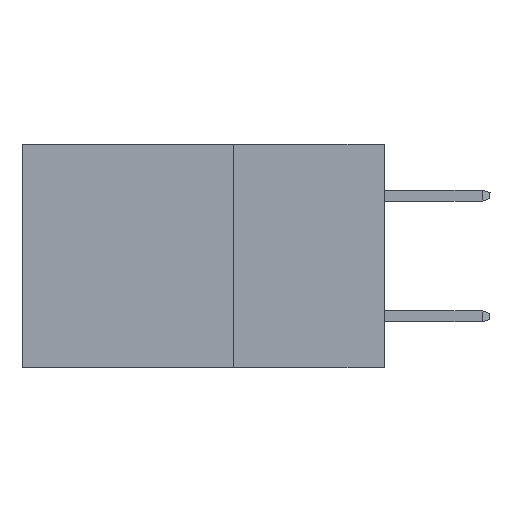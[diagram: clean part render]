
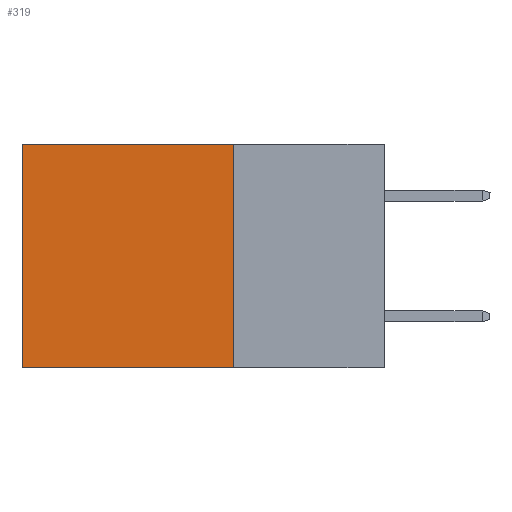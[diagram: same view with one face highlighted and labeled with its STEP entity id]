
A CAD part, left-side view. The second image highlights one B-rep face of the part: STEP entity #319.
In plain terms, the highlighted planar face has unit normal (-1, 0, 0).
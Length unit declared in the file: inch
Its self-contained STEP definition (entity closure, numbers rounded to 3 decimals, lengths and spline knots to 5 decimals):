
#319 = ADVANCED_FACE ( 'NONE', ( #1471 ), #5878, .F. ) ;
#1410 = ORIENTED_EDGE ( 'NONE', *, *, #8651, .T. ) ;
#1471 = FACE_OUTER_BOUND ( 'NONE', #7726, .T. ) ;
#1713 = DIRECTION ( 'NONE',  ( 0., 1., 0. ) ) ;
#1745 = CARTESIAN_POINT ( 'NONE',  ( 0.298, 0.6, 0. ) ) ;
#1840 = VERTEX_POINT ( 'NONE', #15833 ) ;
#2898 = DIRECTION ( 'NONE',  ( 0., 0., -1. ) ) ;
#5604 = CARTESIAN_POINT ( 'NONE',  ( 0.298, 0.25, 0. ) ) ;
#5878 = PLANE ( 'NONE',  #18901 ) ;
#6263 = CARTESIAN_POINT ( 'NONE',  ( 0.298, 0.25, -0.37 ) ) ;
#7000 = ORIENTED_EDGE ( 'NONE', *, *, #9492, .F. ) ;
#7726 = EDGE_LOOP ( 'NONE', ( #1410, #15751, #7000, #14764 ) ) ;
#7983 = VERTEX_POINT ( 'NONE', #20382 ) ;
#8651 = EDGE_CURVE ( 'NONE', #12386, #1840, #10512, .T. ) ;
#9492 = EDGE_CURVE ( 'NONE', #22242, #7983, #14454, .T. ) ;
#9864 = VECTOR ( 'NONE', #2898, 39.37008 ) ;
#10021 = LINE ( 'NONE', #18814, #10562 ) ;
#10512 = LINE ( 'NONE', #1745, #16757 ) ;
#10562 = VECTOR ( 'NONE', #20774, 39.37008 ) ;
#10763 = VECTOR ( 'NONE', #1713, 39.37008 ) ;
#10998 = CARTESIAN_POINT ( 'NONE',  ( 0.298, 0.6, 0. ) ) ;
#11555 = LINE ( 'NONE', #6263, #10763 ) ;
#12386 = VERTEX_POINT ( 'NONE', #10998 ) ;
#12815 = DIRECTION ( 'NONE',  ( 1., 0., 0. ) ) ;
#14454 = LINE ( 'NONE', #18619, #9864 ) ;
#14764 = ORIENTED_EDGE ( 'NONE', *, *, #18802, .T. ) ;
#15751 = ORIENTED_EDGE ( 'NONE', *, *, #21056, .F. ) ;
#15833 = CARTESIAN_POINT ( 'NONE',  ( 0.298, 0.6, -0.37 ) ) ;
#16757 = VECTOR ( 'NONE', #18838, 39.37008 ) ;
#17701 = DIRECTION ( 'NONE',  ( 0., 0., -1. ) ) ;
#18619 = CARTESIAN_POINT ( 'NONE',  ( 0.298, 0.25, 0. ) ) ;
#18802 = EDGE_CURVE ( 'NONE', #22242, #12386, #10021, .T. ) ;
#18814 = CARTESIAN_POINT ( 'NONE',  ( 0.298, 0.25, 0. ) ) ;
#18838 = DIRECTION ( 'NONE',  ( 0., 0., -1. ) ) ;
#18901 = AXIS2_PLACEMENT_3D ( 'NONE', #5604, #12815, #17701 ) ;
#19927 = CARTESIAN_POINT ( 'NONE',  ( 0.298, 0.25, 0. ) ) ;
#20382 = CARTESIAN_POINT ( 'NONE',  ( 0.298, 0.25, -0.37 ) ) ;
#20774 = DIRECTION ( 'NONE',  ( 0., 1., 0. ) ) ;
#21056 = EDGE_CURVE ( 'NONE', #7983, #1840, #11555, .T. ) ;
#22242 = VERTEX_POINT ( 'NONE', #19927 ) ;
